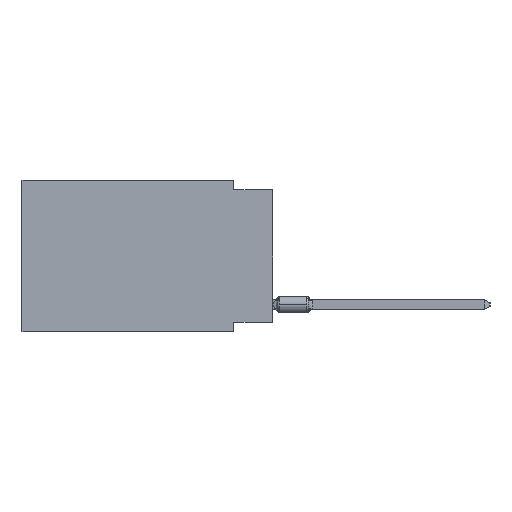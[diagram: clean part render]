
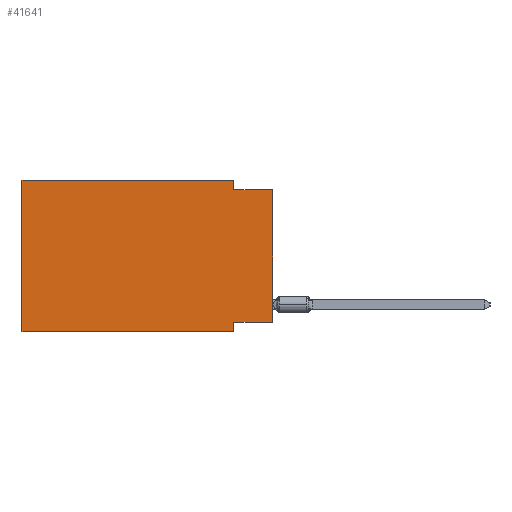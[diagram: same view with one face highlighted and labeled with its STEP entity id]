
A CAD part, left-side view. The second image highlights one B-rep face of the part: STEP entity #41641.
In plain terms, the highlighted planar face has unit normal (-1, 0, 0).
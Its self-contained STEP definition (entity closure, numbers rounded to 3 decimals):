
#2118 = CARTESIAN_POINT ( 'NONE',  ( 0., 0., 0. ) ) ;
#2221 = ORIENTED_EDGE ( 'NONE', *, *, #12805, .F. ) ;
#3774 = CARTESIAN_POINT ( 'NONE',  ( 0., 16.383, 0. ) ) ;
#3860 = CARTESIAN_POINT ( 'NONE',  ( 0., 2.54, -9.906 ) ) ;
#5335 = ORIENTED_EDGE ( 'NONE', *, *, #8854, .F. ) ;
#5770 = LINE ( 'NONE', #59671, #40177 ) ;
#6741 = DIRECTION ( 'NONE',  ( 0., -1., 0. ) ) ;
#7568 = DIRECTION ( 'NONE',  ( 0., 0., 1. ) ) ;
#7962 = VECTOR ( 'NONE', #28733, 1000. ) ;
#8594 = FACE_OUTER_BOUND ( 'NONE', #20262, .T. ) ;
#8854 = EDGE_CURVE ( 'NONE', #16440, #54597, #13496, .T. ) ;
#9010 = DIRECTION ( 'NONE',  ( 0., -1., 0. ) ) ;
#10976 = EDGE_CURVE ( 'NONE', #46779, #13847, #5770, .T. ) ;
#11576 = VERTEX_POINT ( 'NONE', #3860 ) ;
#12174 = CARTESIAN_POINT ( 'NONE',  ( 0., 0., -0.635 ) ) ;
#12612 = EDGE_CURVE ( 'NONE', #46779, #14503, #22314, .T. ) ;
#12685 = CARTESIAN_POINT ( 'NONE',  ( 0., 2.54, 0. ) ) ;
#12805 = EDGE_CURVE ( 'NONE', #13847, #11576, #53107, .T. ) ;
#13081 = VECTOR ( 'NONE', #7568, 1000. ) ;
#13496 = LINE ( 'NONE', #37265, #60400 ) ;
#13847 = VERTEX_POINT ( 'NONE', #43321 ) ;
#14375 = EDGE_CURVE ( 'NONE', #53691, #16440, #19462, .T. ) ;
#14503 = VERTEX_POINT ( 'NONE', #36757 ) ;
#16440 = VERTEX_POINT ( 'NONE', #39623 ) ;
#17919 = CARTESIAN_POINT ( 'NONE',  ( 0., 2.54, 0. ) ) ;
#19462 = LINE ( 'NONE', #58932, #42079 ) ;
#20262 = EDGE_LOOP ( 'NONE', ( #40423, #63029, #30178, #5335, #32938, #40000, #2221, #52212 ) ) ;
#20419 = DIRECTION ( 'NONE',  ( 0., 0., -1. ) ) ;
#20448 = EDGE_CURVE ( 'NONE', #53691, #11576, #40713, .T. ) ;
#22314 = LINE ( 'NONE', #2118, #13081 ) ;
#23868 = EDGE_CURVE ( 'NONE', #59559, #14503, #36577, .T. ) ;
#25953 = DIRECTION ( 'NONE',  ( 0., 1., 0. ) ) ;
#27773 = CARTESIAN_POINT ( 'NONE',  ( 0., 2.54, -9.906 ) ) ;
#28156 = PLANE ( 'NONE',  #40902 ) ;
#28733 = DIRECTION ( 'NONE',  ( 0., 0., -1. ) ) ;
#30178 = ORIENTED_EDGE ( 'NONE', *, *, #57356, .F. ) ;
#30429 = DIRECTION ( 'NONE',  ( 0., -1., 0. ) ) ;
#31370 = CARTESIAN_POINT ( 'NONE',  ( 0., 16.383, -9.906 ) ) ;
#32262 = DIRECTION ( 'NONE',  ( 0., 0., -1. ) ) ;
#32938 = ORIENTED_EDGE ( 'NONE', *, *, #14375, .F. ) ;
#35026 = CARTESIAN_POINT ( 'NONE',  ( 0., 0., -9.271 ) ) ;
#36577 = LINE ( 'NONE', #12174, #45856 ) ;
#36757 = CARTESIAN_POINT ( 'NONE',  ( 0., 0., -0.635 ) ) ;
#37265 = CARTESIAN_POINT ( 'NONE',  ( 0., 16.383, 0. ) ) ;
#37343 = VECTOR ( 'NONE', #30429, 1000. ) ;
#39623 = CARTESIAN_POINT ( 'NONE',  ( 0., 16.383, 0. ) ) ;
#40000 = ORIENTED_EDGE ( 'NONE', *, *, #20448, .T. ) ;
#40177 = VECTOR ( 'NONE', #25953, 1000. ) ;
#40423 = ORIENTED_EDGE ( 'NONE', *, *, #12612, .T. ) ;
#40713 = LINE ( 'NONE', #31370, #37343 ) ;
#40902 = AXIS2_PLACEMENT_3D ( 'NONE', #3774, #62488, #20419 ) ;
#41641 = ADVANCED_FACE ( 'NONE', ( #8594 ), #28156, .F. ) ;
#42079 = VECTOR ( 'NONE', #59571, 1000. ) ;
#43321 = CARTESIAN_POINT ( 'NONE',  ( 0., 2.54, -9.271 ) ) ;
#43425 = VECTOR ( 'NONE', #32262, 1000. ) ;
#45856 = VECTOR ( 'NONE', #6741, 1000. ) ;
#46779 = VERTEX_POINT ( 'NONE', #35026 ) ;
#50571 = CARTESIAN_POINT ( 'NONE',  ( 0., 16.383, -9.906 ) ) ;
#52212 = ORIENTED_EDGE ( 'NONE', *, *, #10976, .F. ) ;
#53107 = LINE ( 'NONE', #27773, #7962 ) ;
#53298 = CARTESIAN_POINT ( 'NONE',  ( 0., 2.54, -0.635 ) ) ;
#53691 = VERTEX_POINT ( 'NONE', #50571 ) ;
#54597 = VERTEX_POINT ( 'NONE', #17919 ) ;
#57356 = EDGE_CURVE ( 'NONE', #54597, #59559, #60521, .T. ) ;
#58932 = CARTESIAN_POINT ( 'NONE',  ( 0., 16.383, 0. ) ) ;
#59559 = VERTEX_POINT ( 'NONE', #53298 ) ;
#59571 = DIRECTION ( 'NONE',  ( 0., 0., 1. ) ) ;
#59671 = CARTESIAN_POINT ( 'NONE',  ( 0., 0., -9.271 ) ) ;
#60400 = VECTOR ( 'NONE', #9010, 1000. ) ;
#60521 = LINE ( 'NONE', #12685, #43425 ) ;
#62488 = DIRECTION ( 'NONE',  ( 1., 0., 0. ) ) ;
#63029 = ORIENTED_EDGE ( 'NONE', *, *, #23868, .F. ) ;
